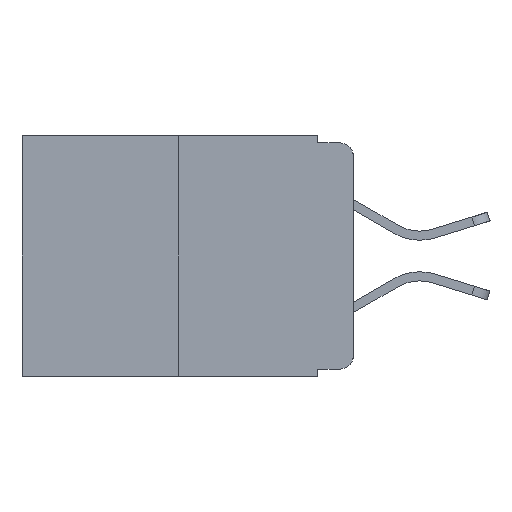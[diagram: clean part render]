
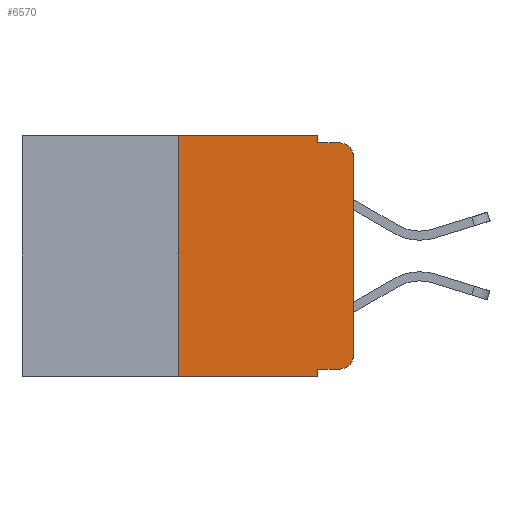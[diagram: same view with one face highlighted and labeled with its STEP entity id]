
A CAD part, left-side view. The second image highlights one B-rep face of the part: STEP entity #6570.
In plain terms, the highlighted planar face has unit normal (-1, 0, 0).
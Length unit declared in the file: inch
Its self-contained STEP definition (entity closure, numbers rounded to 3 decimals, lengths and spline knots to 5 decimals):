
#471 = ORIENTED_EDGE ( 'NONE', *, *, #11741, .T. ) ;
#1321 = CARTESIAN_POINT ( 'NONE',  ( 0., 0., 0. ) ) ;
#1448 = DIRECTION ( 'NONE',  ( 0., 0., -1. ) ) ;
#1752 = LINE ( 'NONE', #7339, #10424 ) ;
#1784 = CARTESIAN_POINT ( 'NONE',  ( 0., 0.051, 0. ) ) ;
#1999 = FACE_OUTER_BOUND ( 'NONE', #9860, .T. ) ;
#2595 = DIRECTION ( 'NONE',  ( 0., 0., 1. ) ) ;
#2737 = DIRECTION ( 'NONE',  ( 0., 0., 1. ) ) ;
#2740 = CARTESIAN_POINT ( 'NONE',  ( 0., 0.051, -0.343 ) ) ;
#3103 = VECTOR ( 'NONE', #4060, 39.37008 ) ;
#3293 = CARTESIAN_POINT ( 'NONE',  ( 0., 0., -0.313 ) ) ;
#3302 = VECTOR ( 'NONE', #12316, 39.37008 ) ;
#3337 = AXIS2_PLACEMENT_3D ( 'NONE', #10206, #3607, #11278 ) ;
#3396 = VERTEX_POINT ( 'NONE', #7931 ) ;
#3427 = VERTEX_POINT ( 'NONE', #5203 ) ;
#3607 = DIRECTION ( 'NONE',  ( -1., 0., 0. ) ) ;
#4060 = DIRECTION ( 'NONE',  ( 0., -1., 0. ) ) ;
#4171 = VERTEX_POINT ( 'NONE', #14339 ) ;
#4175 = CARTESIAN_POINT ( 'NONE',  ( 0., 0.25, -0.343 ) ) ;
#4195 = DIRECTION ( 'NONE',  ( -1., 0., 0. ) ) ;
#4341 = ORIENTED_EDGE ( 'NONE', *, *, #9570, .F. ) ;
#4366 = ORIENTED_EDGE ( 'NONE', *, *, #7449, .T. ) ;
#4598 = VERTEX_POINT ( 'NONE', #10138 ) ;
#4766 = VECTOR ( 'NONE', #2595, 39.37008 ) ;
#5122 = LINE ( 'NONE', #1321, #4766 ) ;
#5203 = CARTESIAN_POINT ( 'NONE',  ( 0., 0., -0.03 ) ) ;
#5303 = CARTESIAN_POINT ( 'NONE',  ( 0., 0.051, 0. ) ) ;
#5855 = CARTESIAN_POINT ( 'NONE',  ( 0., 0.051, -0.333 ) ) ;
#5953 = ORIENTED_EDGE ( 'NONE', *, *, #8160, .F. ) ;
#6197 = LINE ( 'NONE', #7386, #3103 ) ;
#6211 = PLANE ( 'NONE',  #12264 ) ;
#6570 = ADVANCED_FACE ( 'NONE', ( #1999 ), #6211, .F. ) ;
#6721 = EDGE_CURVE ( 'NONE', #4598, #9023, #14428, .T. ) ;
#6781 = VERTEX_POINT ( 'NONE', #1784 ) ;
#6868 = CIRCLE ( 'NONE', #3337, 0.02 ) ;
#7051 = CARTESIAN_POINT ( 'NONE',  ( 0., 0.051, -0.01 ) ) ;
#7326 = CARTESIAN_POINT ( 'NONE',  ( 0., 0.473, 0. ) ) ;
#7339 = CARTESIAN_POINT ( 'NONE',  ( 0., 0.25, 0. ) ) ;
#7386 = CARTESIAN_POINT ( 'NONE',  ( 0., 0.473, 0. ) ) ;
#7442 = VECTOR ( 'NONE', #10580, 39.37008 ) ;
#7449 = EDGE_CURVE ( 'NONE', #11576, #4598, #12858, .T. ) ;
#7931 = CARTESIAN_POINT ( 'NONE',  ( 0., 0.051, -0.01 ) ) ;
#8160 = EDGE_CURVE ( 'NONE', #11576, #10520, #10270, .T. ) ;
#8264 = CARTESIAN_POINT ( 'NONE',  ( 0., 0.25, 0. ) ) ;
#8315 = ORIENTED_EDGE ( 'NONE', *, *, #9478, .F. ) ;
#8395 = DIRECTION ( 'NONE',  ( 1., 0., 0. ) ) ;
#8850 = EDGE_CURVE ( 'NONE', #9819, #9310, #1752, .T. ) ;
#9023 = VERTEX_POINT ( 'NONE', #3293 ) ;
#9209 = LINE ( 'NONE', #7051, #3302 ) ;
#9310 = VERTEX_POINT ( 'NONE', #8264 ) ;
#9415 = ORIENTED_EDGE ( 'NONE', *, *, #11023, .T. ) ;
#9478 = EDGE_CURVE ( 'NONE', #9310, #6781, #6197, .T. ) ;
#9570 = EDGE_CURVE ( 'NONE', #6781, #3396, #11243, .T. ) ;
#9632 = ORIENTED_EDGE ( 'NONE', *, *, #8850, .F. ) ;
#9805 = ORIENTED_EDGE ( 'NONE', *, *, #12802, .T. ) ;
#9819 = VERTEX_POINT ( 'NONE', #4175 ) ;
#9860 = EDGE_LOOP ( 'NONE', ( #471, #9415, #10786, #4341, #8315, #9632, #9805, #5953, #4366, #14147 ) ) ;
#10031 = LINE ( 'NONE', #13960, #12472 ) ;
#10138 = CARTESIAN_POINT ( 'NONE',  ( 0., 0.02, -0.333 ) ) ;
#10206 = CARTESIAN_POINT ( 'NONE',  ( 0., 0.02, -0.03 ) ) ;
#10270 = LINE ( 'NONE', #10523, #7442 ) ;
#10298 = EDGE_CURVE ( 'NONE', #3396, #4171, #9209, .T. ) ;
#10424 = VECTOR ( 'NONE', #2737, 39.37008 ) ;
#10520 = VERTEX_POINT ( 'NONE', #2740 ) ;
#10523 = CARTESIAN_POINT ( 'NONE',  ( 0., 0.051, 0. ) ) ;
#10580 = DIRECTION ( 'NONE',  ( 0., 0., -1. ) ) ;
#10718 = CARTESIAN_POINT ( 'NONE',  ( 0., 0.051, -0.333 ) ) ;
#10737 = CARTESIAN_POINT ( 'NONE',  ( 0., 0.02, -0.313 ) ) ;
#10786 = ORIENTED_EDGE ( 'NONE', *, *, #10298, .F. ) ;
#11023 = EDGE_CURVE ( 'NONE', #3427, #4171, #6868, .T. ) ;
#11243 = LINE ( 'NONE', #5303, #13281 ) ;
#11278 = DIRECTION ( 'NONE',  ( 0., 0., -1. ) ) ;
#11576 = VERTEX_POINT ( 'NONE', #5855 ) ;
#11741 = EDGE_CURVE ( 'NONE', #9023, #3427, #5122, .T. ) ;
#11773 = DIRECTION ( 'NONE',  ( 0., -1., 0. ) ) ;
#11788 = DIRECTION ( 'NONE',  ( 0., 0., -1. ) ) ;
#12264 = AXIS2_PLACEMENT_3D ( 'NONE', #7326, #8395, #1448 ) ;
#12316 = DIRECTION ( 'NONE',  ( 0., -1., 0. ) ) ;
#12472 = VECTOR ( 'NONE', #12956, 39.37008 ) ;
#12554 = VECTOR ( 'NONE', #11773, 39.37008 ) ;
#12802 = EDGE_CURVE ( 'NONE', #9819, #10520, #10031, .T. ) ;
#12858 = LINE ( 'NONE', #10718, #12554 ) ;
#12956 = DIRECTION ( 'NONE',  ( 0., -1., 0. ) ) ;
#13281 = VECTOR ( 'NONE', #13760, 39.37008 ) ;
#13624 = AXIS2_PLACEMENT_3D ( 'NONE', #10737, #4195, #11788 ) ;
#13760 = DIRECTION ( 'NONE',  ( 0., 0., -1. ) ) ;
#13960 = CARTESIAN_POINT ( 'NONE',  ( 0., 0.473, -0.343 ) ) ;
#14147 = ORIENTED_EDGE ( 'NONE', *, *, #6721, .T. ) ;
#14339 = CARTESIAN_POINT ( 'NONE',  ( 0., 0.02, -0.01 ) ) ;
#14428 = CIRCLE ( 'NONE', #13624, 0.02 ) ;
